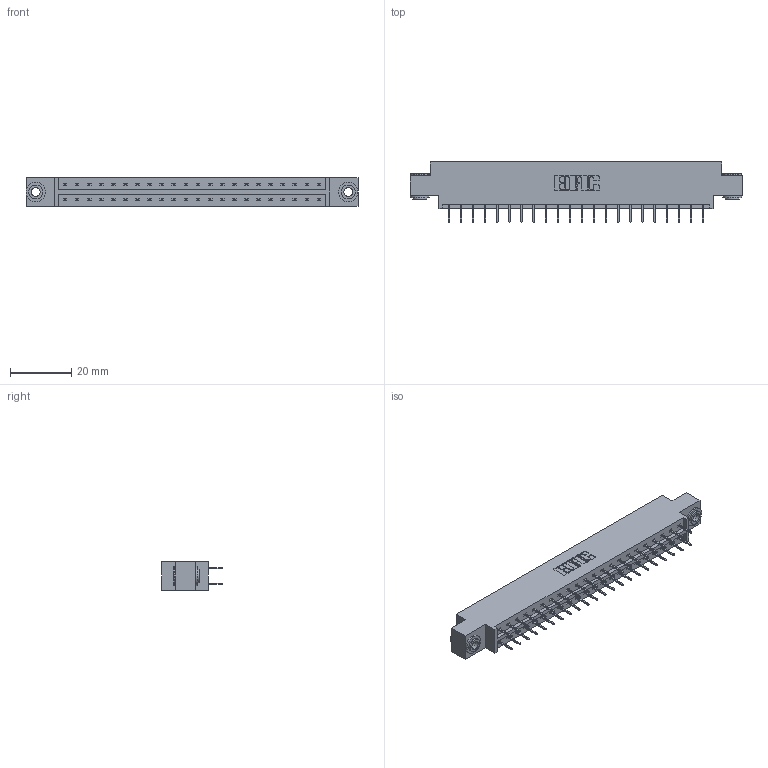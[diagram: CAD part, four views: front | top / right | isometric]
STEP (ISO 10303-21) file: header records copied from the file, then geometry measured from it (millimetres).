
FILE_DESCRIPTION (( 'STEP AP203' ), '1' );
FILE_NAME ('333-044-524-803.STEP', '2018-08-03T21:09:13', ( '' ), ( '' ), 'SwSTEP 2.0', 'SolidWorks 2016', '' );
FILE_SCHEMA (( 'CONFIG_CONTROL_DESIGN' ));
Length unit declared in the file: inch
Products named in the file (4): 333 Part_Offset - .156 Dia - TH; 345-292-001_345-293-124; 345-250-002_345-250-002-102; 333-044-524-803
Assembly tree (47 placements, depth 2):
  333-044-524-803
    333 Part_Offset - .156 Dia - TH
    345-292-001_345-293-124  x44
    345-250-002_345-250-002-102  x2
Bounding box: 108.71 x 19.69 x 9.4 mm (x, y, z)
Volume: 10636.9 mm3; surface area: 12602.4 mm2
Topology: 47 solids, 47 shells, 2620 faces, 7395 edges, 4750 vertices
Faces by surface type: plane 1932, cylinder 680, cone 8
Entity records: 17596 total; most frequent: CARTESIAN_POINT 2917, ORIENTED_EDGE 2846, DIRECTION 2561, EDGE_CURVE 1423, VECTOR 1275, LINE 1275, VERTEX_POINT 942, AXIS2_PLACEMENT_3D 643
